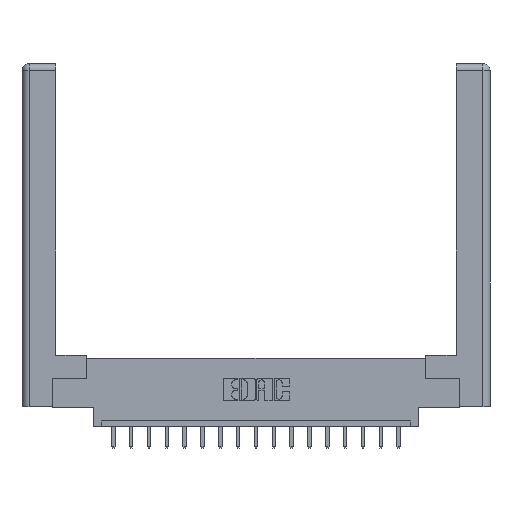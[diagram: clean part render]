
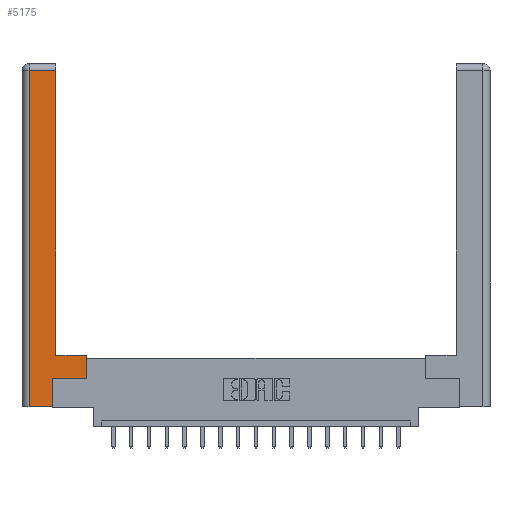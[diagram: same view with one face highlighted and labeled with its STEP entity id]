
A CAD part, top view. The second image highlights one B-rep face of the part: STEP entity #5175.
In plain terms, the highlighted planar face has unit normal (0, 0, 1).
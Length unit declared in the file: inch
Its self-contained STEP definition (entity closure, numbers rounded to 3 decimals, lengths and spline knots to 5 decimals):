
#311 = VERTEX_POINT ( 'NONE', #927 ) ;
#350 = LINE ( 'NONE', #5504, #15507 ) ;
#927 = CARTESIAN_POINT ( 'NONE',  ( 0.295, 0.45, 0. ) ) ;
#1390 = DIRECTION ( 'NONE',  ( -1., 0., 0. ) ) ;
#1930 = DIRECTION ( 'NONE',  ( -1., 0., 0. ) ) ;
#2102 = LINE ( 'NONE', #9334, #17962 ) ;
#2241 = EDGE_CURVE ( 'NONE', #8376, #15693, #350, .T. ) ;
#3033 = ORIENTED_EDGE ( 'NONE', *, *, #12438, .T. ) ;
#3183 = CARTESIAN_POINT ( 'NONE',  ( 0.295, 3., 0. ) ) ;
#4159 = VECTOR ( 'NONE', #5118, 39.37008 ) ;
#5118 = DIRECTION ( 'NONE',  ( -1., 0., 0. ) ) ;
#5175 = ADVANCED_FACE ( 'NONE', ( #5303 ), #10709, .F. ) ;
#5181 = ORIENTED_EDGE ( 'NONE', *, *, #12319, .T. ) ;
#5206 = CARTESIAN_POINT ( 'NONE',  ( 0.295, 2.94, 0. ) ) ;
#5238 = CARTESIAN_POINT ( 'NONE',  ( 0.565, 0.245, 0. ) ) ;
#5303 = FACE_OUTER_BOUND ( 'NONE', #12278, .T. ) ;
#5504 = CARTESIAN_POINT ( 'NONE',  ( 0.0615, 2.94, 0. ) ) ;
#5872 = VERTEX_POINT ( 'NONE', #5238 ) ;
#6097 = LINE ( 'NONE', #7337, #14467 ) ;
#6230 = DIRECTION ( 'NONE',  ( 0., 1., 0. ) ) ;
#6779 = VECTOR ( 'NONE', #7320, 39.37008 ) ;
#7197 = CARTESIAN_POINT ( 'NONE',  ( 0.0615, 0., 0. ) ) ;
#7320 = DIRECTION ( 'NONE',  ( 0., 1., 0. ) ) ;
#7337 = CARTESIAN_POINT ( 'NONE',  ( 0.265, 0.245, 0. ) ) ;
#7627 = ORIENTED_EDGE ( 'NONE', *, *, #18433, .T. ) ;
#7816 = CARTESIAN_POINT ( 'NONE',  ( 0.265, 0., 0. ) ) ;
#7879 = DIRECTION ( 'NONE',  ( 1., 0., 0. ) ) ;
#8002 = LINE ( 'NONE', #10755, #4159 ) ;
#8376 = VERTEX_POINT ( 'NONE', #5206 ) ;
#8626 = CARTESIAN_POINT ( 'NONE',  ( 0.265, 0.245, 0. ) ) ;
#8664 = CARTESIAN_POINT ( 'NONE',  ( 0.0615, 0., 0. ) ) ;
#8872 = EDGE_CURVE ( 'NONE', #311, #8376, #16915, .T. ) ;
#9334 = CARTESIAN_POINT ( 'NONE',  ( 0.565, 0.245, 0. ) ) ;
#9986 = AXIS2_PLACEMENT_3D ( 'NONE', #16408, #10648, #1930 ) ;
#10137 = DIRECTION ( 'NONE',  ( 0., -1., 0. ) ) ;
#10430 = VERTEX_POINT ( 'NONE', #8626 ) ;
#10648 = DIRECTION ( 'NONE',  ( 0., 0., -1. ) ) ;
#10709 = PLANE ( 'NONE',  #9986 ) ;
#10755 = CARTESIAN_POINT ( 'NONE',  ( 0.295, 0.45, 0. ) ) ;
#11190 = VERTEX_POINT ( 'NONE', #18061 ) ;
#11688 = VECTOR ( 'NONE', #6230, 39.37008 ) ;
#11889 = EDGE_CURVE ( 'NONE', #5872, #11190, #15159, .T. ) ;
#12278 = EDGE_LOOP ( 'NONE', ( #18753, #12771, #5181, #7627, #3033, #13644, #18669, #14333 ) ) ;
#12319 = EDGE_CURVE ( 'NONE', #15693, #18139, #14926, .T. ) ;
#12438 = EDGE_CURVE ( 'NONE', #15246, #10430, #6097, .T. ) ;
#12628 = VECTOR ( 'NONE', #17774, 39.37008 ) ;
#12771 = ORIENTED_EDGE ( 'NONE', *, *, #2241, .T. ) ;
#13105 = CARTESIAN_POINT ( 'NONE',  ( 0.565, 0.45, 0. ) ) ;
#13115 = VECTOR ( 'NONE', #10137, 39.37008 ) ;
#13588 = CARTESIAN_POINT ( 'NONE',  ( 0.265, 0., 0. ) ) ;
#13644 = ORIENTED_EDGE ( 'NONE', *, *, #15569, .T. ) ;
#14333 = ORIENTED_EDGE ( 'NONE', *, *, #14933, .T. ) ;
#14467 = VECTOR ( 'NONE', #14631, 39.37008 ) ;
#14631 = DIRECTION ( 'NONE',  ( 0., 1., 0. ) ) ;
#14926 = LINE ( 'NONE', #8664, #13115 ) ;
#14933 = EDGE_CURVE ( 'NONE', #11190, #311, #8002, .T. ) ;
#15159 = LINE ( 'NONE', #13105, #6779 ) ;
#15246 = VERTEX_POINT ( 'NONE', #13588 ) ;
#15507 = VECTOR ( 'NONE', #1390, 39.37008 ) ;
#15569 = EDGE_CURVE ( 'NONE', #10430, #5872, #2102, .T. ) ;
#15693 = VERTEX_POINT ( 'NONE', #17003 ) ;
#16408 = CARTESIAN_POINT ( 'NONE',  ( 0., 0., 0. ) ) ;
#16915 = LINE ( 'NONE', #3183, #11688 ) ;
#17003 = CARTESIAN_POINT ( 'NONE',  ( 0.0615, 2.94, 0. ) ) ;
#17375 = LINE ( 'NONE', #7816, #12628 ) ;
#17774 = DIRECTION ( 'NONE',  ( 1., 0., 0. ) ) ;
#17962 = VECTOR ( 'NONE', #7879, 39.37008 ) ;
#18061 = CARTESIAN_POINT ( 'NONE',  ( 0.565, 0.45, 0. ) ) ;
#18139 = VERTEX_POINT ( 'NONE', #7197 ) ;
#18433 = EDGE_CURVE ( 'NONE', #18139, #15246, #17375, .T. ) ;
#18669 = ORIENTED_EDGE ( 'NONE', *, *, #11889, .T. ) ;
#18753 = ORIENTED_EDGE ( 'NONE', *, *, #8872, .T. ) ;
